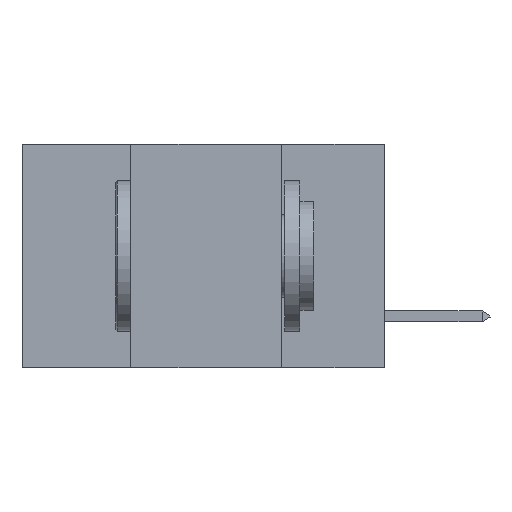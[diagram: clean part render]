
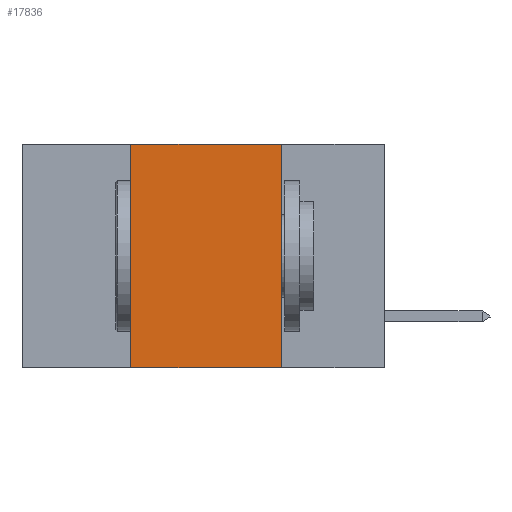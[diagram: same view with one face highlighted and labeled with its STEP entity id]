
A CAD part, left-side view. The second image highlights one B-rep face of the part: STEP entity #17836.
In plain terms, the highlighted planar face has unit normal (-1, 0, 0).
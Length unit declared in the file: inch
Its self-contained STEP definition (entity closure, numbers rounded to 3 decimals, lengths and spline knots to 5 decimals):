
#184 = EDGE_CURVE ( 'NONE', #5920, #9865, #17873, .T. ) ;
#757 = VECTOR ( 'NONE', #13365, 39.37008 ) ;
#1042 = DIRECTION ( 'NONE',  ( 0., 0., -1. ) ) ;
#1067 = ORIENTED_EDGE ( 'NONE', *, *, #184, .F. ) ;
#1350 = CARTESIAN_POINT ( 'NONE',  ( 0., 0.6, -0.37 ) ) ;
#2762 = VECTOR ( 'NONE', #14210, 39.37008 ) ;
#2882 = CARTESIAN_POINT ( 'NONE',  ( 0., 0.17, -0.37 ) ) ;
#3753 = ORIENTED_EDGE ( 'NONE', *, *, #17137, .F. ) ;
#3970 = CARTESIAN_POINT ( 'NONE',  ( 0., 0.6, 0. ) ) ;
#4449 = LINE ( 'NONE', #1350, #7381 ) ;
#4637 = LINE ( 'NONE', #10456, #757 ) ;
#5319 = ORIENTED_EDGE ( 'NONE', *, *, #17320, .T. ) ;
#5920 = VERTEX_POINT ( 'NONE', #12738 ) ;
#6400 = CARTESIAN_POINT ( 'NONE',  ( 0., 0.42, 0. ) ) ;
#7381 = VECTOR ( 'NONE', #20172, 39.37008 ) ;
#9865 = VERTEX_POINT ( 'NONE', #14117 ) ;
#10456 = CARTESIAN_POINT ( 'NONE',  ( 0., 0.17, 0. ) ) ;
#11909 = DIRECTION ( 'NONE',  ( 1., 0., 0. ) ) ;
#12392 = EDGE_LOOP ( 'NONE', ( #15762, #1067, #3753, #5319 ) ) ;
#12738 = CARTESIAN_POINT ( 'NONE',  ( 0., 0.42, 0. ) ) ;
#13233 = LINE ( 'NONE', #6400, #2762 ) ;
#13365 = DIRECTION ( 'NONE',  ( 0., 0., -1. ) ) ;
#13624 = CARTESIAN_POINT ( 'NONE',  ( 0., 0.42, -0.37 ) ) ;
#14117 = CARTESIAN_POINT ( 'NONE',  ( 0., 0.17, 0. ) ) ;
#14210 = DIRECTION ( 'NONE',  ( 0., 0., 1. ) ) ;
#14874 = AXIS2_PLACEMENT_3D ( 'NONE', #16293, #11909, #1042 ) ;
#15762 = ORIENTED_EDGE ( 'NONE', *, *, #18683, .F. ) ;
#16132 = FACE_OUTER_BOUND ( 'NONE', #12392, .T. ) ;
#16293 = CARTESIAN_POINT ( 'NONE',  ( 0., 0.6, 0. ) ) ;
#17137 = EDGE_CURVE ( 'NONE', #19091, #5920, #13233, .T. ) ;
#17320 = EDGE_CURVE ( 'NONE', #19091, #17436, #4449, .T. ) ;
#17436 = VERTEX_POINT ( 'NONE', #2882 ) ;
#17836 = ADVANCED_FACE ( 'NONE', ( #16132 ), #19363, .F. ) ;
#17873 = LINE ( 'NONE', #3970, #19833 ) ;
#18683 = EDGE_CURVE ( 'NONE', #9865, #17436, #4637, .T. ) ;
#19091 = VERTEX_POINT ( 'NONE', #13624 ) ;
#19363 = PLANE ( 'NONE',  #14874 ) ;
#19573 = DIRECTION ( 'NONE',  ( 0., -1., 0. ) ) ;
#19833 = VECTOR ( 'NONE', #19573, 39.37008 ) ;
#20172 = DIRECTION ( 'NONE',  ( 0., -1., 0. ) ) ;
